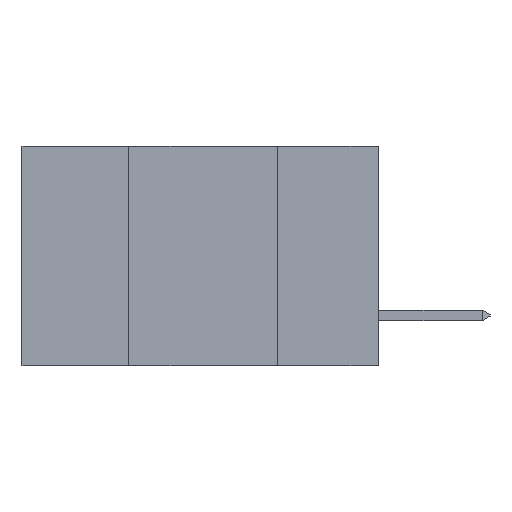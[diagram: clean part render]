
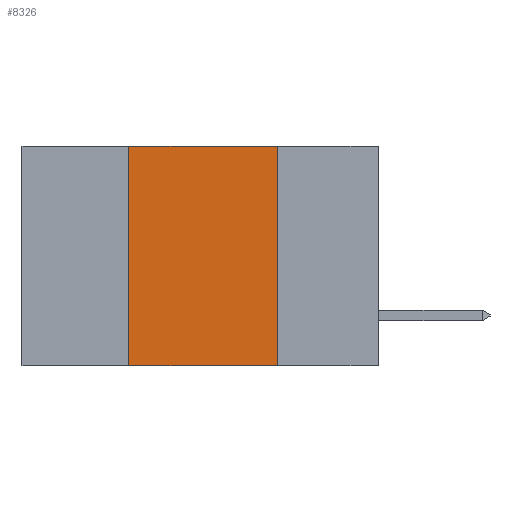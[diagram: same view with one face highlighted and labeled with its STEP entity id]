
A CAD part, left-side view. The second image highlights one B-rep face of the part: STEP entity #8326.
In plain terms, the highlighted planar face has unit normal (-1, 0, 0).
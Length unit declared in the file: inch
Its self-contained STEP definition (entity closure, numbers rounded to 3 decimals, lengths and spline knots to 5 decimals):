
#174 = PLANE ( 'NONE',  #10632 ) ;
#382 = LINE ( 'NONE', #11689, #7506 ) ;
#1619 = DIRECTION ( 'NONE',  ( 1., 0., 0. ) ) ;
#2143 = EDGE_CURVE ( 'NONE', #2468, #9044, #15379, .T. ) ;
#2468 = VERTEX_POINT ( 'NONE', #6284 ) ;
#2915 = DIRECTION ( 'NONE',  ( 0., -1., 0. ) ) ;
#2930 = CARTESIAN_POINT ( 'NONE',  ( 0., 0.6, -0.37 ) ) ;
#3200 = DIRECTION ( 'NONE',  ( 0., -1., 0. ) ) ;
#3289 = DIRECTION ( 'NONE',  ( 0., 0., -1. ) ) ;
#4179 = LINE ( 'NONE', #14139, #7468 ) ;
#6284 = CARTESIAN_POINT ( 'NONE',  ( 0., 0.42, -0.37 ) ) ;
#6939 = CARTESIAN_POINT ( 'NONE',  ( 0., 0.42, 0. ) ) ;
#7468 = VECTOR ( 'NONE', #2915, 39.37008 ) ;
#7506 = VECTOR ( 'NONE', #3289, 39.37008 ) ;
#8162 = VERTEX_POINT ( 'NONE', #6939 ) ;
#8326 = ADVANCED_FACE ( 'NONE', ( #14652 ), #174, .F. ) ;
#9044 = VERTEX_POINT ( 'NONE', #15493 ) ;
#9528 = EDGE_LOOP ( 'NONE', ( #9892, #14045, #17772, #11641 ) ) ;
#9892 = ORIENTED_EDGE ( 'NONE', *, *, #15360, .F. ) ;
#10147 = VECTOR ( 'NONE', #11042, 39.37008 ) ;
#10632 = AXIS2_PLACEMENT_3D ( 'NONE', #17060, #1619, #11469 ) ;
#11042 = DIRECTION ( 'NONE',  ( 0., 0., 1. ) ) ;
#11469 = DIRECTION ( 'NONE',  ( 0., 0., -1. ) ) ;
#11581 = EDGE_CURVE ( 'NONE', #2468, #8162, #17589, .T. ) ;
#11632 = VECTOR ( 'NONE', #3200, 39.37008 ) ;
#11641 = ORIENTED_EDGE ( 'NONE', *, *, #2143, .T. ) ;
#11689 = CARTESIAN_POINT ( 'NONE',  ( 0., 0.17, -0.37 ) ) ;
#12449 = CARTESIAN_POINT ( 'NONE',  ( 0., 0.42, -0.37 ) ) ;
#13442 = EDGE_CURVE ( 'NONE', #8162, #13496, #4179, .T. ) ;
#13496 = VERTEX_POINT ( 'NONE', #15683 ) ;
#14045 = ORIENTED_EDGE ( 'NONE', *, *, #13442, .F. ) ;
#14139 = CARTESIAN_POINT ( 'NONE',  ( 0., 0.6, 0. ) ) ;
#14652 = FACE_OUTER_BOUND ( 'NONE', #9528, .T. ) ;
#15360 = EDGE_CURVE ( 'NONE', #13496, #9044, #382, .T. ) ;
#15379 = LINE ( 'NONE', #2930, #11632 ) ;
#15493 = CARTESIAN_POINT ( 'NONE',  ( 0., 0.17, -0.37 ) ) ;
#15683 = CARTESIAN_POINT ( 'NONE',  ( 0., 0.17, 0. ) ) ;
#17060 = CARTESIAN_POINT ( 'NONE',  ( 0., 0.6, 0. ) ) ;
#17589 = LINE ( 'NONE', #12449, #10147 ) ;
#17772 = ORIENTED_EDGE ( 'NONE', *, *, #11581, .F. ) ;
